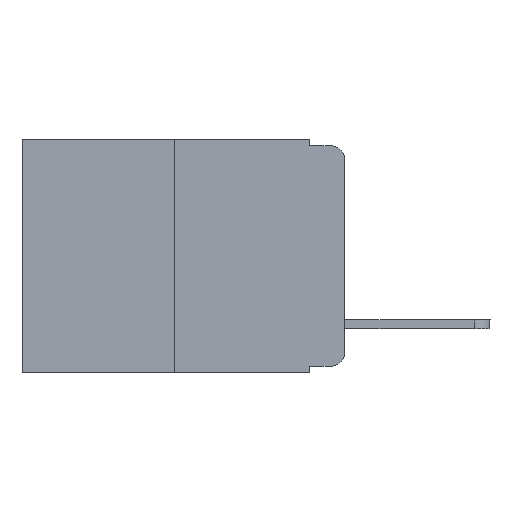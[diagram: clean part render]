
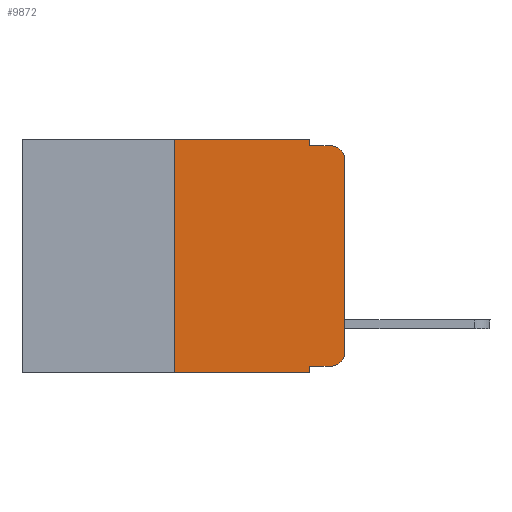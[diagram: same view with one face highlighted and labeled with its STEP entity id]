
A CAD part, left-side view. The second image highlights one B-rep face of the part: STEP entity #9872.
In plain terms, the highlighted planar face has unit normal (-1, 0, 0).
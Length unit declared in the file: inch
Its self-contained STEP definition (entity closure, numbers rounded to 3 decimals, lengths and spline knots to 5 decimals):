
#297 = EDGE_CURVE ( 'NONE', #1567, #8160, #3799, .T. ) ;
#324 = ORIENTED_EDGE ( 'NONE', *, *, #9876, .F. ) ;
#413 = CARTESIAN_POINT ( 'NONE',  ( 0., 0.051, -0.333 ) ) ;
#454 = DIRECTION ( 'NONE',  ( 0., -1., 0. ) ) ;
#483 = LINE ( 'NONE', #4480, #2995 ) ;
#556 = DIRECTION ( 'NONE',  ( 0., 0., 1. ) ) ;
#588 = CARTESIAN_POINT ( 'NONE',  ( 0., 0.051, -0.01 ) ) ;
#630 = PLANE ( 'NONE',  #4958 ) ;
#937 = CARTESIAN_POINT ( 'NONE',  ( 0., 0.02, -0.313 ) ) ;
#969 = DIRECTION ( 'NONE',  ( -1., 0., 0. ) ) ;
#976 = DIRECTION ( 'NONE',  ( 0., 0., -1. ) ) ;
#1153 = ORIENTED_EDGE ( 'NONE', *, *, #10206, .T. ) ;
#1489 = DIRECTION ( 'NONE',  ( 0., 0., 1. ) ) ;
#1558 = ORIENTED_EDGE ( 'NONE', *, *, #3487, .F. ) ;
#1567 = VERTEX_POINT ( 'NONE', #2651 ) ;
#1886 = VECTOR ( 'NONE', #2017, 39.37008 ) ;
#1959 = EDGE_CURVE ( 'NONE', #5678, #2625, #7090, .T. ) ;
#2017 = DIRECTION ( 'NONE',  ( 0., 0., -1. ) ) ;
#2164 = FACE_OUTER_BOUND ( 'NONE', #2808, .T. ) ;
#2625 = VERTEX_POINT ( 'NONE', #8625 ) ;
#2651 = CARTESIAN_POINT ( 'NONE',  ( 0., 0.02, -0.333 ) ) ;
#2786 = VERTEX_POINT ( 'NONE', #5182 ) ;
#2808 = EDGE_LOOP ( 'NONE', ( #10555, #1153, #5013, #1558, #324, #11709, #4720, #2975, #11696, #8124 ) ) ;
#2975 = ORIENTED_EDGE ( 'NONE', *, *, #10941, .F. ) ;
#2995 = VECTOR ( 'NONE', #3614, 39.37008 ) ;
#3204 = DIRECTION ( 'NONE',  ( 0., 0., -1. ) ) ;
#3487 = EDGE_CURVE ( 'NONE', #7515, #5678, #10918, .T. ) ;
#3593 = CIRCLE ( 'NONE', #6779, 0.02 ) ;
#3614 = DIRECTION ( 'NONE',  ( 0., -1., 0. ) ) ;
#3799 = CIRCLE ( 'NONE', #5043, 0.02 ) ;
#4052 = CARTESIAN_POINT ( 'NONE',  ( 0., 0., -0.313 ) ) ;
#4168 = CARTESIAN_POINT ( 'NONE',  ( 0., 0., 0. ) ) ;
#4236 = CARTESIAN_POINT ( 'NONE',  ( 0., 0.473, 0. ) ) ;
#4356 = CARTESIAN_POINT ( 'NONE',  ( 0., 0.25, 0. ) ) ;
#4480 = CARTESIAN_POINT ( 'NONE',  ( 0., 0.473, -0.343 ) ) ;
#4720 = ORIENTED_EDGE ( 'NONE', *, *, #9315, .T. ) ;
#4958 = AXIS2_PLACEMENT_3D ( 'NONE', #8773, #10598, #6983 ) ;
#4998 = CARTESIAN_POINT ( 'NONE',  ( 0., 0.051, 0. ) ) ;
#5013 = ORIENTED_EDGE ( 'NONE', *, *, #1959, .F. ) ;
#5036 = DIRECTION ( 'NONE',  ( 0., -1., 0. ) ) ;
#5043 = AXIS2_PLACEMENT_3D ( 'NONE', #937, #969, #7343 ) ;
#5070 = CARTESIAN_POINT ( 'NONE',  ( 0., 0.051, -0.343 ) ) ;
#5182 = CARTESIAN_POINT ( 'NONE',  ( 0., 0.25, 0. ) ) ;
#5503 = DIRECTION ( 'NONE',  ( -1., 0., 0. ) ) ;
#5678 = VERTEX_POINT ( 'NONE', #588 ) ;
#5803 = VECTOR ( 'NONE', #556, 39.37008 ) ;
#5900 = CARTESIAN_POINT ( 'NONE',  ( 0., 0.051, -0.01 ) ) ;
#6025 = CARTESIAN_POINT ( 'NONE',  ( 0., 0.051, 0. ) ) ;
#6085 = VERTEX_POINT ( 'NONE', #7461 ) ;
#6451 = LINE ( 'NONE', #4236, #7452 ) ;
#6554 = CARTESIAN_POINT ( 'NONE',  ( 0., 0.25, -0.343 ) ) ;
#6779 = AXIS2_PLACEMENT_3D ( 'NONE', #10984, #5503, #976 ) ;
#6983 = DIRECTION ( 'NONE',  ( 0., 0., -1. ) ) ;
#7007 = EDGE_CURVE ( 'NONE', #8160, #6085, #9091, .T. ) ;
#7090 = LINE ( 'NONE', #5900, #9982 ) ;
#7343 = DIRECTION ( 'NONE',  ( 0., 0., -1. ) ) ;
#7365 = CARTESIAN_POINT ( 'NONE',  ( 0., 0.051, -0.333 ) ) ;
#7452 = VECTOR ( 'NONE', #10634, 39.37008 ) ;
#7461 = CARTESIAN_POINT ( 'NONE',  ( 0., 0., -0.03 ) ) ;
#7515 = VERTEX_POINT ( 'NONE', #6025 ) ;
#7744 = LINE ( 'NONE', #413, #9762 ) ;
#8030 = LINE ( 'NONE', #9365, #1886 ) ;
#8124 = ORIENTED_EDGE ( 'NONE', *, *, #297, .T. ) ;
#8160 = VERTEX_POINT ( 'NONE', #4052 ) ;
#8483 = VECTOR ( 'NONE', #3204, 39.37008 ) ;
#8530 = EDGE_CURVE ( 'NONE', #9349, #2786, #11177, .T. ) ;
#8625 = CARTESIAN_POINT ( 'NONE',  ( 0., 0.02, -0.01 ) ) ;
#8773 = CARTESIAN_POINT ( 'NONE',  ( 0., 0.473, 0. ) ) ;
#9091 = LINE ( 'NONE', #4168, #5803 ) ;
#9315 = EDGE_CURVE ( 'NONE', #9349, #9852, #483, .T. ) ;
#9349 = VERTEX_POINT ( 'NONE', #6554 ) ;
#9365 = CARTESIAN_POINT ( 'NONE',  ( 0., 0.051, 0. ) ) ;
#9595 = EDGE_CURVE ( 'NONE', #10800, #1567, #7744, .T. ) ;
#9762 = VECTOR ( 'NONE', #454, 39.37008 ) ;
#9852 = VERTEX_POINT ( 'NONE', #5070 ) ;
#9872 = ADVANCED_FACE ( 'NONE', ( #2164 ), #630, .F. ) ;
#9876 = EDGE_CURVE ( 'NONE', #2786, #7515, #6451, .T. ) ;
#9982 = VECTOR ( 'NONE', #5036, 39.37008 ) ;
#10074 = VECTOR ( 'NONE', #1489, 39.37008 ) ;
#10206 = EDGE_CURVE ( 'NONE', #6085, #2625, #3593, .T. ) ;
#10555 = ORIENTED_EDGE ( 'NONE', *, *, #7007, .T. ) ;
#10598 = DIRECTION ( 'NONE',  ( 1., 0., 0. ) ) ;
#10634 = DIRECTION ( 'NONE',  ( 0., -1., 0. ) ) ;
#10800 = VERTEX_POINT ( 'NONE', #7365 ) ;
#10918 = LINE ( 'NONE', #4998, #8483 ) ;
#10941 = EDGE_CURVE ( 'NONE', #10800, #9852, #8030, .T. ) ;
#10984 = CARTESIAN_POINT ( 'NONE',  ( 0., 0.02, -0.03 ) ) ;
#11177 = LINE ( 'NONE', #4356, #10074 ) ;
#11696 = ORIENTED_EDGE ( 'NONE', *, *, #9595, .T. ) ;
#11709 = ORIENTED_EDGE ( 'NONE', *, *, #8530, .F. ) ;
